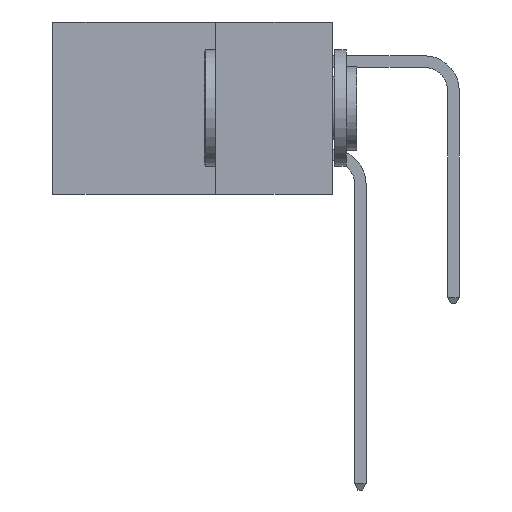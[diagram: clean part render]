
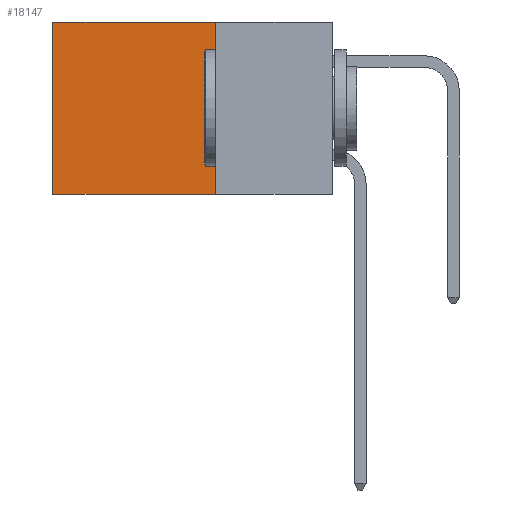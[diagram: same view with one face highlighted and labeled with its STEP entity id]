
A CAD part, left-side view. The second image highlights one B-rep face of the part: STEP entity #18147.
In plain terms, the highlighted planar face has unit normal (-1, 0, 0).
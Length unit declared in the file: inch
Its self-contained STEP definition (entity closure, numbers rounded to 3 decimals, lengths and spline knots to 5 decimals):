
#200 = ORIENTED_EDGE ( 'NONE', *, *, #6120, .F. ) ;
#266 = ORIENTED_EDGE ( 'NONE', *, *, #9004, .T. ) ;
#803 = PLANE ( 'NONE',  #14712 ) ;
#1819 = CARTESIAN_POINT ( 'NONE',  ( 0.2615, 0.25, -0.37 ) ) ;
#2527 = ORIENTED_EDGE ( 'NONE', *, *, #19724, .T. ) ;
#2914 = VECTOR ( 'NONE', #14867, 39.37008 ) ;
#3090 = DIRECTION ( 'NONE',  ( 1., 0., 0. ) ) ;
#4088 = VECTOR ( 'NONE', #5386, 39.37008 ) ;
#4820 = CARTESIAN_POINT ( 'NONE',  ( 0.2615, 0.25, -0.37 ) ) ;
#5092 = EDGE_LOOP ( 'NONE', ( #266, #200, #9732, #2527 ) ) ;
#5386 = DIRECTION ( 'NONE',  ( 0., 0., -1. ) ) ;
#5774 = LINE ( 'NONE', #20915, #27860 ) ;
#6120 = EDGE_CURVE ( 'NONE', #11641, #17962, #5774, .T. ) ;
#9004 = EDGE_CURVE ( 'NONE', #16295, #17962, #21198, .T. ) ;
#9411 = LINE ( 'NONE', #1819, #2914 ) ;
#9732 = ORIENTED_EDGE ( 'NONE', *, *, #25947, .F. ) ;
#9860 = CARTESIAN_POINT ( 'NONE',  ( 0.2615, 0.25, 0. ) ) ;
#11024 = LINE ( 'NONE', #9860, #21026 ) ;
#11641 = VERTEX_POINT ( 'NONE', #16082 ) ;
#14005 = CARTESIAN_POINT ( 'NONE',  ( 0.2615, 0.6, -0.37 ) ) ;
#14712 = AXIS2_PLACEMENT_3D ( 'NONE', #4820, #3090, #18121 ) ;
#14799 = FACE_OUTER_BOUND ( 'NONE', #5092, .T. ) ;
#14867 = DIRECTION ( 'NONE',  ( 0., 0., -1. ) ) ;
#16082 = CARTESIAN_POINT ( 'NONE',  ( 0.2615, 0.25, -0.37 ) ) ;
#16295 = VERTEX_POINT ( 'NONE', #22767 ) ;
#17962 = VERTEX_POINT ( 'NONE', #23620 ) ;
#18121 = DIRECTION ( 'NONE',  ( 0., 0., -1. ) ) ;
#18147 = ADVANCED_FACE ( 'NONE', ( #14799 ), #803, .F. ) ;
#19724 = EDGE_CURVE ( 'NONE', #27709, #16295, #11024, .T. ) ;
#20549 = DIRECTION ( 'NONE',  ( 0., 1., 0. ) ) ;
#20915 = CARTESIAN_POINT ( 'NONE',  ( 0.2615, 0.25, -0.37 ) ) ;
#21026 = VECTOR ( 'NONE', #20549, 39.37008 ) ;
#21198 = LINE ( 'NONE', #14005, #4088 ) ;
#22767 = CARTESIAN_POINT ( 'NONE',  ( 0.2615, 0.6, 0. ) ) ;
#23437 = CARTESIAN_POINT ( 'NONE',  ( 0.2615, 0.25, 0. ) ) ;
#23620 = CARTESIAN_POINT ( 'NONE',  ( 0.2615, 0.6, -0.37 ) ) ;
#25226 = DIRECTION ( 'NONE',  ( 0., 1., 0. ) ) ;
#25947 = EDGE_CURVE ( 'NONE', #27709, #11641, #9411, .T. ) ;
#27709 = VERTEX_POINT ( 'NONE', #23437 ) ;
#27860 = VECTOR ( 'NONE', #25226, 39.37008 ) ;
